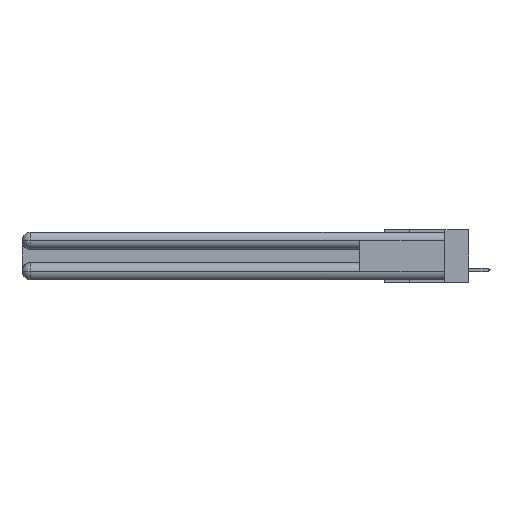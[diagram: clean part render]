
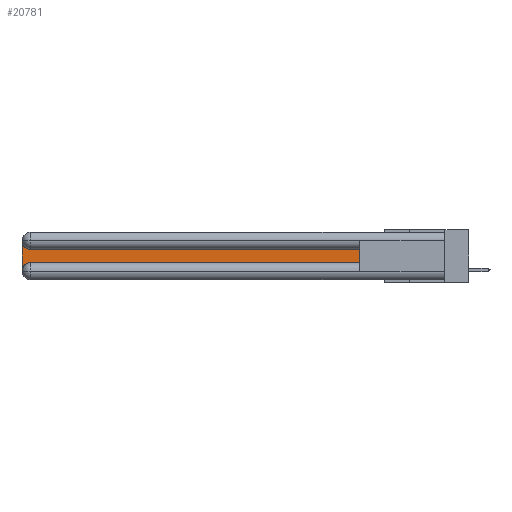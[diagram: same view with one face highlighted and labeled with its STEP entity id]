
A CAD part, left-side view. The second image highlights one B-rep face of the part: STEP entity #20781.
In plain terms, the highlighted planar face has unit normal (-1, 0, 0).
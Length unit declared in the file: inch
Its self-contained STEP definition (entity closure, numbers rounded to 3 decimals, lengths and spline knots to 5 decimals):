
#647 = CARTESIAN_POINT ( 'NONE',  ( 0.075, 3., -0.2175 ) ) ;
#953 = VECTOR ( 'NONE', #23907, 39.37008 ) ;
#1446 = CARTESIAN_POINT ( 'NONE',  ( 0.075, 0.6, -0.2175 ) ) ;
#1620 = ORIENTED_EDGE ( 'NONE', *, *, #26212, .T. ) ;
#2434 = DIRECTION ( 'NONE',  ( 1., 0., 0. ) ) ;
#2823 = DIRECTION ( 'NONE',  ( 0., 0., 1. ) ) ;
#3135 = CARTESIAN_POINT ( 'NONE',  ( 0.075, 2.94, -0.2175 ) ) ;
#3862 = VECTOR ( 'NONE', #17639, 39.37008 ) ;
#5071 = CARTESIAN_POINT ( 'NONE',  ( 0.075, 0.6, -0.2175 ) ) ;
#5077 = EDGE_CURVE ( 'NONE', #23546, #10380, #18213, .T. ) ;
#5199 = EDGE_LOOP ( 'NONE', ( #20612, #21766, #6461, #1620, #11836, #6592 ) ) ;
#5951 = VERTEX_POINT ( 'NONE', #3135 ) ;
#6442 = LINE ( 'NONE', #647, #953 ) ;
#6448 = VECTOR ( 'NONE', #19192, 39.37008 ) ;
#6461 = ORIENTED_EDGE ( 'NONE', *, *, #19731, .T. ) ;
#6592 = ORIENTED_EDGE ( 'NONE', *, *, #15405, .T. ) ;
#6669 = CARTESIAN_POINT ( 'NONE',  ( 0.075, 2.94, -0.1225 ) ) ;
#8231 = PLANE ( 'NONE',  #11902 ) ;
#8583 = CARTESIAN_POINT ( 'NONE',  ( 0.075, 2.94, -0.0625 ) ) ;
#8889 = CARTESIAN_POINT ( 'NONE',  ( 0.075, 3., -0.0625 ) ) ;
#9176 = CIRCLE ( 'NONE', #18350, 0.06 ) ;
#9579 = VERTEX_POINT ( 'NONE', #1446 ) ;
#9674 = LINE ( 'NONE', #24229, #3862 ) ;
#10380 = VERTEX_POINT ( 'NONE', #8889 ) ;
#10458 = DIRECTION ( 'NONE',  ( 1., 0., 0. ) ) ;
#10748 = VERTEX_POINT ( 'NONE', #16220 ) ;
#10876 = FACE_OUTER_BOUND ( 'NONE', #5199, .T. ) ;
#11645 = EDGE_CURVE ( 'NONE', #5951, #9579, #22852, .T. ) ;
#11836 = ORIENTED_EDGE ( 'NONE', *, *, #11645, .T. ) ;
#11902 = AXIS2_PLACEMENT_3D ( 'NONE', #14530, #10458, #21164 ) ;
#12668 = VECTOR ( 'NONE', #2823, 39.37008 ) ;
#14530 = CARTESIAN_POINT ( 'NONE',  ( 0.075, 3., -0.1225 ) ) ;
#15356 = DIRECTION ( 'NONE',  ( 0., 0., -1. ) ) ;
#15405 = EDGE_CURVE ( 'NONE', #9579, #10748, #19751, .T. ) ;
#16220 = CARTESIAN_POINT ( 'NONE',  ( 0.075, 0.6, -0.1225 ) ) ;
#17639 = DIRECTION ( 'NONE',  ( 0., 1., 0. ) ) ;
#18213 = CIRCLE ( 'NONE', #25110, 0.06 ) ;
#18350 = AXIS2_PLACEMENT_3D ( 'NONE', #18405, #18688, #15356 ) ;
#18405 = CARTESIAN_POINT ( 'NONE',  ( 0.075, 2.94, -0.2775 ) ) ;
#18563 = CARTESIAN_POINT ( 'NONE',  ( 0.075, 0.6, -0.2175 ) ) ;
#18688 = DIRECTION ( 'NONE',  ( 1., 0., 0. ) ) ;
#18907 = DIRECTION ( 'NONE',  ( 0., 0., -1. ) ) ;
#19192 = DIRECTION ( 'NONE',  ( 0., -1., 0. ) ) ;
#19277 = VERTEX_POINT ( 'NONE', #21709 ) ;
#19325 = EDGE_CURVE ( 'NONE', #10748, #23546, #9674, .T. ) ;
#19731 = EDGE_CURVE ( 'NONE', #10380, #19277, #6442, .T. ) ;
#19751 = LINE ( 'NONE', #5071, #12668 ) ;
#20612 = ORIENTED_EDGE ( 'NONE', *, *, #19325, .T. ) ;
#20781 = ADVANCED_FACE ( 'NONE', ( #10876 ), #8231, .F. ) ;
#21164 = DIRECTION ( 'NONE',  ( 0., 0., -1. ) ) ;
#21709 = CARTESIAN_POINT ( 'NONE',  ( 0.075, 3., -0.2775 ) ) ;
#21766 = ORIENTED_EDGE ( 'NONE', *, *, #5077, .T. ) ;
#22852 = LINE ( 'NONE', #18563, #6448 ) ;
#23546 = VERTEX_POINT ( 'NONE', #6669 ) ;
#23907 = DIRECTION ( 'NONE',  ( 0., 0., -1. ) ) ;
#24229 = CARTESIAN_POINT ( 'NONE',  ( 0.075, 0.6, -0.1225 ) ) ;
#25110 = AXIS2_PLACEMENT_3D ( 'NONE', #8583, #2434, #18907 ) ;
#26212 = EDGE_CURVE ( 'NONE', #19277, #5951, #9176, .T. ) ;
